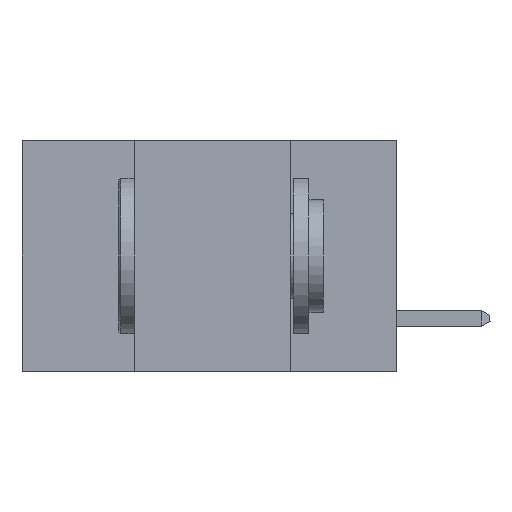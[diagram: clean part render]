
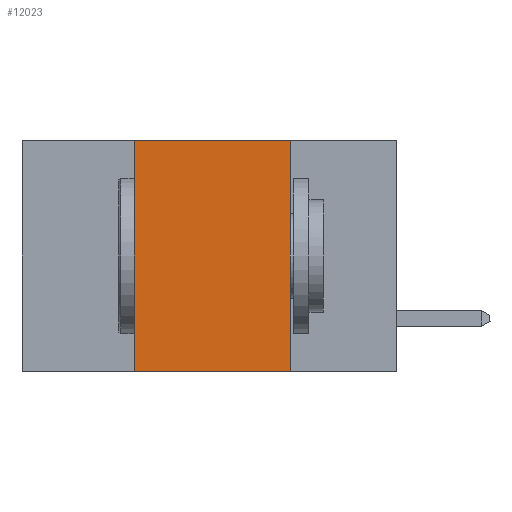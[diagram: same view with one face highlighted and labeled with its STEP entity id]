
A CAD part, left-side view. The second image highlights one B-rep face of the part: STEP entity #12023.
In plain terms, the highlighted planar face has unit normal (-1, 0, 0).
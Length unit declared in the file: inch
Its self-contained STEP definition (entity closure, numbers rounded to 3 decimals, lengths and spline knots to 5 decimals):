
#92 = CARTESIAN_POINT ( 'NONE',  ( 0., 0.42, -0.37 ) ) ;
#576 = ORIENTED_EDGE ( 'NONE', *, *, #28638, .F. ) ;
#1739 = DIRECTION ( 'NONE',  ( 1., 0., 0. ) ) ;
#2500 = AXIS2_PLACEMENT_3D ( 'NONE', #19846, #1739, #6266 ) ;
#4191 = CARTESIAN_POINT ( 'NONE',  ( 0., 0.17, 0. ) ) ;
#4275 = ORIENTED_EDGE ( 'NONE', *, *, #19856, .F. ) ;
#5121 = VERTEX_POINT ( 'NONE', #18903 ) ;
#5471 = CARTESIAN_POINT ( 'NONE',  ( 0., 0.42, 0. ) ) ;
#5488 = CARTESIAN_POINT ( 'NONE',  ( 0., 0.6, -0.37 ) ) ;
#6266 = DIRECTION ( 'NONE',  ( 0., 0., -1. ) ) ;
#6547 = CARTESIAN_POINT ( 'NONE',  ( 0., 0.17, 0. ) ) ;
#6700 = VECTOR ( 'NONE', #21349, 39.37008 ) ;
#8543 = VECTOR ( 'NONE', #21378, 39.37008 ) ;
#8964 = CARTESIAN_POINT ( 'NONE',  ( 0., 0.6, 0. ) ) ;
#9083 = VERTEX_POINT ( 'NONE', #26292 ) ;
#10895 = PLANE ( 'NONE',  #2500 ) ;
#12023 = ADVANCED_FACE ( 'NONE', ( #17692 ), #10895, .F. ) ;
#13056 = EDGE_CURVE ( 'NONE', #14558, #9083, #29203, .T. ) ;
#14558 = VERTEX_POINT ( 'NONE', #92 ) ;
#15810 = EDGE_LOOP ( 'NONE', ( #17037, #576, #4275, #20122 ) ) ;
#17037 = ORIENTED_EDGE ( 'NONE', *, *, #28464, .F. ) ;
#17692 = FACE_OUTER_BOUND ( 'NONE', #15810, .T. ) ;
#18903 = CARTESIAN_POINT ( 'NONE',  ( 0., 0.42, 0. ) ) ;
#19846 = CARTESIAN_POINT ( 'NONE',  ( 0., 0.6, 0. ) ) ;
#19856 = EDGE_CURVE ( 'NONE', #14558, #5121, #28767, .T. ) ;
#19900 = DIRECTION ( 'NONE',  ( 0., 0., -1. ) ) ;
#20122 = ORIENTED_EDGE ( 'NONE', *, *, #13056, .T. ) ;
#20187 = DIRECTION ( 'NONE',  ( 0., -1., 0. ) ) ;
#21349 = DIRECTION ( 'NONE',  ( 0., 0., 1. ) ) ;
#21378 = DIRECTION ( 'NONE',  ( 0., -1., 0. ) ) ;
#23502 = LINE ( 'NONE', #4191, #26388 ) ;
#26047 = VECTOR ( 'NONE', #20187, 39.37008 ) ;
#26292 = CARTESIAN_POINT ( 'NONE',  ( 0., 0.17, -0.37 ) ) ;
#26388 = VECTOR ( 'NONE', #19900, 39.37008 ) ;
#27475 = VERTEX_POINT ( 'NONE', #6547 ) ;
#28464 = EDGE_CURVE ( 'NONE', #27475, #9083, #23502, .T. ) ;
#28638 = EDGE_CURVE ( 'NONE', #5121, #27475, #29267, .T. ) ;
#28767 = LINE ( 'NONE', #5471, #6700 ) ;
#29203 = LINE ( 'NONE', #5488, #8543 ) ;
#29267 = LINE ( 'NONE', #8964, #26047 ) ;
